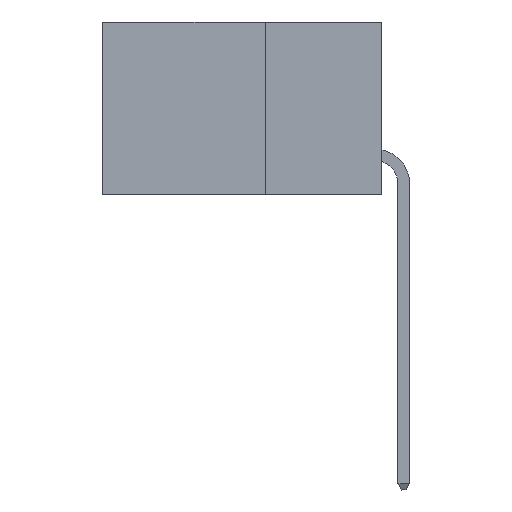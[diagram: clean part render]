
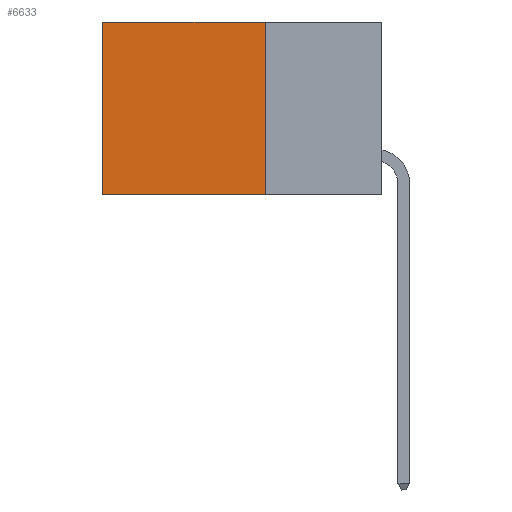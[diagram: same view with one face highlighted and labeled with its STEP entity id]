
A CAD part, left-side view. The second image highlights one B-rep face of the part: STEP entity #6633.
In plain terms, the highlighted planar face has unit normal (-1, 0, 0).
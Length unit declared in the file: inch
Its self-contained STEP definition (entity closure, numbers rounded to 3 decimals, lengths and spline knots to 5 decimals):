
#302 = DIRECTION ( 'NONE',  ( 0., 1., 0. ) ) ;
#369 = CARTESIAN_POINT ( 'NONE',  ( 0.2875, 0.25, -0.37 ) ) ;
#482 = VERTEX_POINT ( 'NONE', #2253 ) ;
#1502 = VECTOR ( 'NONE', #1807, 39.37008 ) ;
#1807 = DIRECTION ( 'NONE',  ( 0., 0., -1. ) ) ;
#2253 = CARTESIAN_POINT ( 'NONE',  ( 0.2875, 0.25, 0. ) ) ;
#2434 = EDGE_CURVE ( 'NONE', #11852, #2828, #7474, .T. ) ;
#2671 = ORIENTED_EDGE ( 'NONE', *, *, #2852, .T. ) ;
#2828 = VERTEX_POINT ( 'NONE', #10453 ) ;
#2852 = EDGE_CURVE ( 'NONE', #482, #11421, #5237, .T. ) ;
#3400 = VECTOR ( 'NONE', #14633, 39.37008 ) ;
#3405 = CARTESIAN_POINT ( 'NONE',  ( 0.2875, 0.25, 0. ) ) ;
#4672 = DIRECTION ( 'NONE',  ( 0., 1., 0. ) ) ;
#4936 = LINE ( 'NONE', #7970, #1502 ) ;
#5101 = AXIS2_PLACEMENT_3D ( 'NONE', #13983, #15140, #8240 ) ;
#5117 = EDGE_CURVE ( 'NONE', #11421, #2828, #4936, .T. ) ;
#5237 = LINE ( 'NONE', #3405, #14153 ) ;
#6633 = ADVANCED_FACE ( 'NONE', ( #10433 ), #7081, .F. ) ;
#7081 = PLANE ( 'NONE',  #5101 ) ;
#7305 = ORIENTED_EDGE ( 'NONE', *, *, #2434, .F. ) ;
#7474 = LINE ( 'NONE', #369, #13266 ) ;
#7970 = CARTESIAN_POINT ( 'NONE',  ( 0.2875, 0.6, 0. ) ) ;
#8240 = DIRECTION ( 'NONE',  ( 0., 0., -1. ) ) ;
#9098 = CARTESIAN_POINT ( 'NONE',  ( 0.2875, 0.25, -0.37 ) ) ;
#9562 = CARTESIAN_POINT ( 'NONE',  ( 0.2875, 0.6, 0. ) ) ;
#10433 = FACE_OUTER_BOUND ( 'NONE', #12391, .T. ) ;
#10453 = CARTESIAN_POINT ( 'NONE',  ( 0.2875, 0.6, -0.37 ) ) ;
#11421 = VERTEX_POINT ( 'NONE', #9562 ) ;
#11548 = ORIENTED_EDGE ( 'NONE', *, *, #15556, .F. ) ;
#11824 = ORIENTED_EDGE ( 'NONE', *, *, #5117, .T. ) ;
#11852 = VERTEX_POINT ( 'NONE', #9098 ) ;
#12391 = EDGE_LOOP ( 'NONE', ( #11824, #7305, #11548, #2671 ) ) ;
#13266 = VECTOR ( 'NONE', #302, 39.37008 ) ;
#13983 = CARTESIAN_POINT ( 'NONE',  ( 0.2875, 0.25, 0. ) ) ;
#14153 = VECTOR ( 'NONE', #4672, 39.37008 ) ;
#14633 = DIRECTION ( 'NONE',  ( 0., 0., -1. ) ) ;
#14683 = CARTESIAN_POINT ( 'NONE',  ( 0.2875, 0.25, 0. ) ) ;
#15140 = DIRECTION ( 'NONE',  ( 1., 0., 0. ) ) ;
#15495 = LINE ( 'NONE', #14683, #3400 ) ;
#15556 = EDGE_CURVE ( 'NONE', #482, #11852, #15495, .T. ) ;
